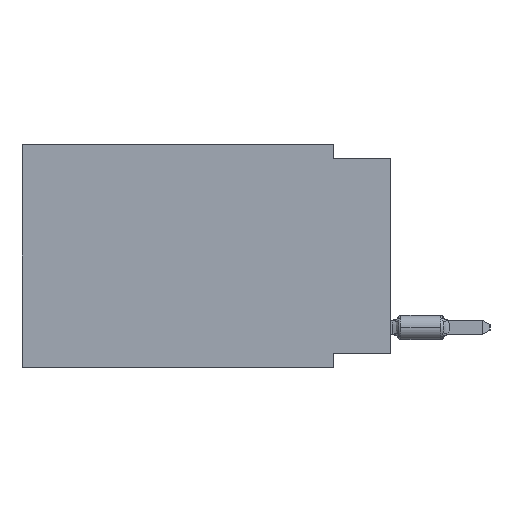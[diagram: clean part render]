
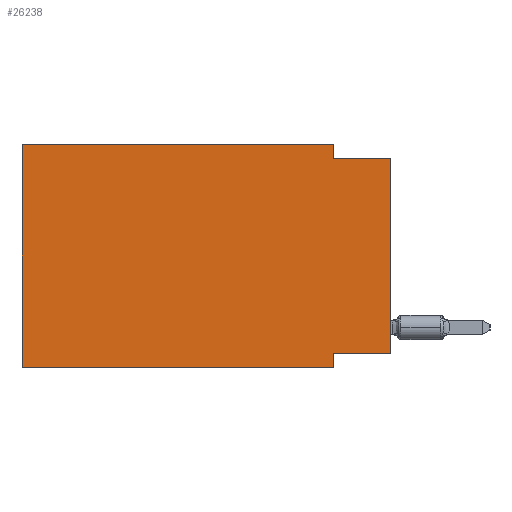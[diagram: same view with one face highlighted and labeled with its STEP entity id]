
A CAD part, left-side view. The second image highlights one B-rep face of the part: STEP entity #26238.
In plain terms, the highlighted planar face has unit normal (-1, 0, 0).
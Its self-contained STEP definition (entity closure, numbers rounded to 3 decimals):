
#2632 = CARTESIAN_POINT ( 'NONE',  ( 0., 2.54, 0. ) ) ;
#2741 = EDGE_CURVE ( 'NONE', #48887, #19484, #20250, .T. ) ;
#4072 = DIRECTION ( 'NONE',  ( 0., 1., 0. ) ) ;
#4359 = DIRECTION ( 'NONE',  ( 0., -1., 0. ) ) ;
#4883 = DIRECTION ( 'NONE',  ( 0., -1., 0. ) ) ;
#4970 = DIRECTION ( 'NONE',  ( 0., 0., -1. ) ) ;
#7911 = ORIENTED_EDGE ( 'NONE', *, *, #17416, .F. ) ;
#10045 = DIRECTION ( 'NONE',  ( 0., -1., 0. ) ) ;
#10119 = VERTEX_POINT ( 'NONE', #25650 ) ;
#11634 = EDGE_CURVE ( 'NONE', #17217, #19484, #39550, .T. ) ;
#12147 = VERTEX_POINT ( 'NONE', #29144 ) ;
#13928 = DIRECTION ( 'NONE',  ( 0., 0., -1. ) ) ;
#14359 = CARTESIAN_POINT ( 'NONE',  ( 0., 16.383, 0. ) ) ;
#16862 = CARTESIAN_POINT ( 'NONE',  ( 0., 16.383, -9.906 ) ) ;
#17192 = CARTESIAN_POINT ( 'NONE',  ( 0., 0., -9.271 ) ) ;
#17217 = VERTEX_POINT ( 'NONE', #17192 ) ;
#17416 = EDGE_CURVE ( 'NONE', #17217, #25038, #46363, .T. ) ;
#18402 = VERTEX_POINT ( 'NONE', #21058 ) ;
#18710 = ORIENTED_EDGE ( 'NONE', *, *, #22186, .F. ) ;
#19484 = VERTEX_POINT ( 'NONE', #46528 ) ;
#20250 = LINE ( 'NONE', #39386, #48806 ) ;
#20327 = VECTOR ( 'NONE', #4970, 1000. ) ;
#20334 = LINE ( 'NONE', #2632, #20327 ) ;
#21058 = CARTESIAN_POINT ( 'NONE',  ( 0., 2.54, 0. ) ) ;
#21156 = LINE ( 'NONE', #16862, #31881 ) ;
#21595 = EDGE_CURVE ( 'NONE', #25038, #38940, #24992, .T. ) ;
#21711 = DIRECTION ( 'NONE',  ( 0., 0., -1. ) ) ;
#22186 = EDGE_CURVE ( 'NONE', #12147, #10119, #25925, .T. ) ;
#22329 = ORIENTED_EDGE ( 'NONE', *, *, #2741, .F. ) ;
#23148 = ORIENTED_EDGE ( 'NONE', *, *, #44906, .F. ) ;
#23422 = EDGE_LOOP ( 'NONE', ( #25875, #22329, #23148, #47501, #18710, #49290, #36450, #7911 ) ) ;
#24992 = LINE ( 'NONE', #37310, #48865 ) ;
#25000 = EDGE_CURVE ( 'NONE', #10119, #18402, #41297, .T. ) ;
#25038 = VERTEX_POINT ( 'NONE', #25926 ) ;
#25650 = CARTESIAN_POINT ( 'NONE',  ( 0., 16.383, 0. ) ) ;
#25713 = VECTOR ( 'NONE', #10045, 1000. ) ;
#25875 = ORIENTED_EDGE ( 'NONE', *, *, #11634, .T. ) ;
#25925 = LINE ( 'NONE', #38003, #27191 ) ;
#25926 = CARTESIAN_POINT ( 'NONE',  ( 0., 2.54, -9.271 ) ) ;
#26238 = ADVANCED_FACE ( 'NONE', ( #32550 ), #48644, .F. ) ;
#27099 = CARTESIAN_POINT ( 'NONE',  ( 0., 2.54, -0.635 ) ) ;
#27191 = VECTOR ( 'NONE', #33735, 1000. ) ;
#29144 = CARTESIAN_POINT ( 'NONE',  ( 0., 16.383, -9.906 ) ) ;
#29279 = CARTESIAN_POINT ( 'NONE',  ( 0., 16.383, 0. ) ) ;
#30333 = VECTOR ( 'NONE', #44291, 1000. ) ;
#31881 = VECTOR ( 'NONE', #4359, 1000. ) ;
#32477 = CARTESIAN_POINT ( 'NONE',  ( 0., 0., 0. ) ) ;
#32550 = FACE_OUTER_BOUND ( 'NONE', #23422, .T. ) ;
#33735 = DIRECTION ( 'NONE',  ( 0., 0., 1. ) ) ;
#33847 = VECTOR ( 'NONE', #4072, 1000. ) ;
#36450 = ORIENTED_EDGE ( 'NONE', *, *, #21595, .F. ) ;
#37310 = CARTESIAN_POINT ( 'NONE',  ( 0., 2.54, -9.906 ) ) ;
#38003 = CARTESIAN_POINT ( 'NONE',  ( 0., 16.383, 0. ) ) ;
#38701 = AXIS2_PLACEMENT_3D ( 'NONE', #29279, #41113, #13928 ) ;
#38940 = VERTEX_POINT ( 'NONE', #46183 ) ;
#39386 = CARTESIAN_POINT ( 'NONE',  ( 0., 0., -0.635 ) ) ;
#39550 = LINE ( 'NONE', #32477, #30333 ) ;
#41113 = DIRECTION ( 'NONE',  ( 1., 0., 0. ) ) ;
#41297 = LINE ( 'NONE', #14359, #25713 ) ;
#43324 = CARTESIAN_POINT ( 'NONE',  ( 0., 0., -9.271 ) ) ;
#44291 = DIRECTION ( 'NONE',  ( 0., 0., 1. ) ) ;
#44906 = EDGE_CURVE ( 'NONE', #18402, #48887, #20334, .T. ) ;
#46183 = CARTESIAN_POINT ( 'NONE',  ( 0., 2.54, -9.906 ) ) ;
#46363 = LINE ( 'NONE', #43324, #33847 ) ;
#46528 = CARTESIAN_POINT ( 'NONE',  ( 0., 0., -0.635 ) ) ;
#46951 = EDGE_CURVE ( 'NONE', #12147, #38940, #21156, .T. ) ;
#47501 = ORIENTED_EDGE ( 'NONE', *, *, #25000, .F. ) ;
#48644 = PLANE ( 'NONE',  #38701 ) ;
#48806 = VECTOR ( 'NONE', #4883, 1000. ) ;
#48865 = VECTOR ( 'NONE', #21711, 1000. ) ;
#48887 = VERTEX_POINT ( 'NONE', #27099 ) ;
#49290 = ORIENTED_EDGE ( 'NONE', *, *, #46951, .T. ) ;
